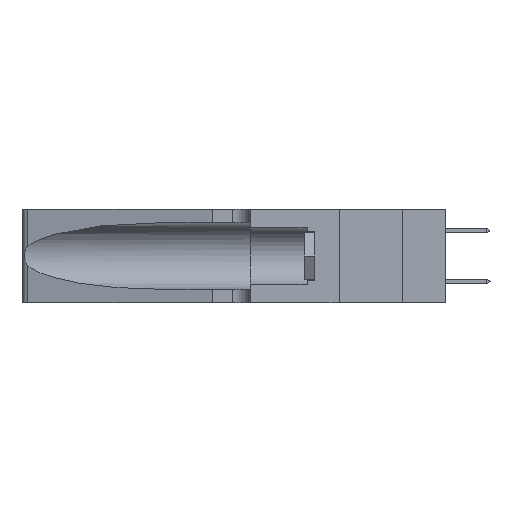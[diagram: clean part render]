
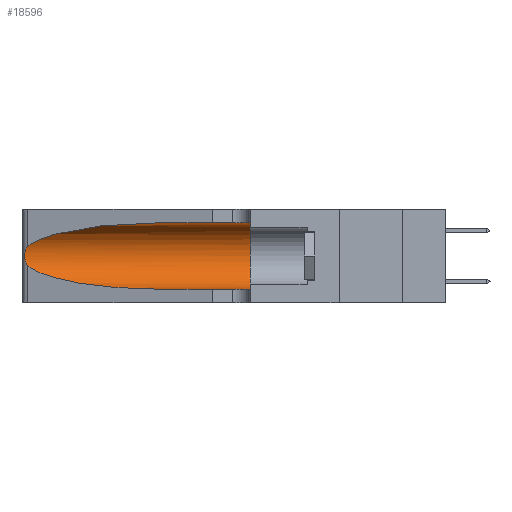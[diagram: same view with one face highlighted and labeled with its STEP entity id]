
A CAD part, left-side view. The second image highlights one B-rep face of the part: STEP entity #18596.
In plain terms, the highlighted cylindrical face has radius 3.308 mm (diameter 6.617 mm), a partial arc.
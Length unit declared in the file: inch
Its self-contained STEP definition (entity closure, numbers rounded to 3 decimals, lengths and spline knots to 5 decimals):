
#35 = AXIS2_PLACEMENT_3D ( 'NONE', #16822, #6896, #2547 ) ;
#482 = CIRCLE ( 'NONE', #35, 0.13025 ) ;
#870 = CARTESIAN_POINT ( 'NONE',  ( 0.25487, 1.22718, 0.14631 ) ) ;
#1161 = VERTEX_POINT ( 'NONE', #9389 ) ;
#1802 = ORIENTED_EDGE ( 'NONE', *, *, #7298, .T. ) ;
#2356 = CARTESIAN_POINT ( 'NONE',  ( 0.18966, 0.96281, 0.31525 ) ) ;
#2547 = DIRECTION ( 'NONE',  ( 0., 0., 1. ) ) ;
#2928 = CARTESIAN_POINT ( 'NONE',  ( 0.25789, 1.23486, 0.15765 ) ) ;
#2979 = CARTESIAN_POINT ( 'NONE',  ( 0.1305, 0.72297, 0.31525 ) ) ;
#3035 = CARTESIAN_POINT ( 'NONE',  ( 0.25487, 1.22718, 0.14631 ) ) ;
#3127 = CYLINDRICAL_SURFACE ( 'NONE', #32522, 0.13025 ) ;
#4473 = CARTESIAN_POINT ( 'NONE',  ( 0.1305, 1.61858, 0.31525 ) ) ;
#5204 = EDGE_CURVE ( 'NONE', #24129, #1161, #13698, .T. ) ;
#5272 = CARTESIAN_POINT ( 'NONE',  ( 0.1305, 0.35, 0.31525 ) ) ;
#5570 = CARTESIAN_POINT ( 'NONE',  ( 0.25639, 1.23184, 0.21858 ) ) ;
#6896 = DIRECTION ( 'NONE',  ( 0., 1., 0. ) ) ;
#7298 = EDGE_CURVE ( 'NONE', #15252, #26612, #16400, .T. ) ;
#7768 = EDGE_CURVE ( 'NONE', #15252, #15232, #14858, .T. ) ;
#7951 = CARTESIAN_POINT ( 'NONE',  ( 0.1305, 0.72297, 0.31525 ) ) ;
#8171 = CARTESIAN_POINT ( 'NONE',  ( 0.25639, 1.23186, 0.15144 ) ) ;
#8453 = CARTESIAN_POINT ( 'NONE',  ( 0.26075, 1.23896, 0.178 ) ) ;
#9302 = DIRECTION ( 'NONE',  ( 0., 0., -1. ) ) ;
#9389 = CARTESIAN_POINT ( 'NONE',  ( 0.1305, 0.35, 0.05475 ) ) ;
#9943 = ORIENTED_EDGE ( 'NONE', *, *, #29032, .T. ) ;
#10994 = CARTESIAN_POINT ( 'NONE',  ( 0.25854, 1.2359, 0.20912 ) ) ;
#11046 = EDGE_CURVE ( 'NONE', #15232, #1161, #482, .T. ) ;
#11238 = CARTESIAN_POINT ( 'NONE',  ( 0.25487, 1.22718, 0.22369 ) ) ;
#11675 = VECTOR ( 'NONE', #27186, 39.37008 ) ;
#11795 = B_SPLINE_CURVE_WITH_KNOTS ( 'NONE', 3,
 ( #13508, #31803, #5570, #21675, #10994, #26729, #24198, #8453, #31702, #15930, #2928, #8171, #29154, #3035 ),
 .UNSPECIFIED., .F., .F.,
 ( 4, 2, 2, 2, 2, 2, 4 ),
 ( 0., 0.00027, 0.00053, 0.00107, 0.0016, 0.00187, 0.00214 ),
 .UNSPECIFIED. ) ;
#12964 = CARTESIAN_POINT ( 'NONE',  ( 0.2373, 1.15595, 0.28018 ) ) ;
#13508 = CARTESIAN_POINT ( 'NONE',  ( 0.25487, 1.22718, 0.22369 ) ) ;
#13698 = LINE ( 'NONE', #13721, #11675 ) ;
#13721 = CARTESIAN_POINT ( 'NONE',  ( 0.1305, 1.61858, 0.05475 ) ) ;
#14858 = LINE ( 'NONE', #4473, #19383 ) ;
#14935 = DIRECTION ( 'NONE',  ( 0., -1., 0. ) ) ;
#14974 =( BOUNDED_CURVE ( )  B_SPLINE_CURVE ( 3, ( #870, #32442, #29368, #21584 ),
 .UNSPECIFIED., .F., .T. ) 
 B_SPLINE_CURVE_WITH_KNOTS ( ( 4, 4 ),
 ( 3.44316, 4.71239 ),
 .UNSPECIFIED. ) 
 CURVE ( )  GEOMETRIC_REPRESENTATION_ITEM ( )  RATIONAL_B_SPLINE_CURVE ( ( 1., 0.87, 0.87, 1. ) ) 
 REPRESENTATION_ITEM ( '' )  );
#15232 = VERTEX_POINT ( 'NONE', #5272 ) ;
#15252 = VERTEX_POINT ( 'NONE', #2979 ) ;
#15535 = FACE_OUTER_BOUND ( 'NONE', #16329, .T. ) ;
#15930 = CARTESIAN_POINT ( 'NONE',  ( 0.25856, 1.23593, 0.16098 ) ) ;
#16329 = EDGE_LOOP ( 'NONE', ( #1802, #9943, #26717, #25968, #26990, #27705 ) ) ;
#16400 =( BOUNDED_CURVE ( )  B_SPLINE_CURVE ( 3, ( #7951, #2356, #12964, #21028 ),
 .UNSPECIFIED., .F., .T. ) 
 B_SPLINE_CURVE_WITH_KNOTS ( ( 4, 4 ),
 ( 1.5708, 2.84003 ),
 .UNSPECIFIED. ) 
 CURVE ( )  GEOMETRIC_REPRESENTATION_ITEM ( )  RATIONAL_B_SPLINE_CURVE ( ( 1., 0.87, 0.87, 1. ) ) 
 REPRESENTATION_ITEM ( '' )  );
#16822 = CARTESIAN_POINT ( 'NONE',  ( 0.1305, 0.35, 0.185 ) ) ;
#18596 = ADVANCED_FACE ( 'NONE', ( #15535 ), #3127, .F. ) ;
#19383 = VECTOR ( 'NONE', #14935, 39.37008 ) ;
#20105 = DIRECTION ( 'NONE',  ( 0., -1., 0. ) ) ;
#21028 = CARTESIAN_POINT ( 'NONE',  ( 0.25487, 1.22718, 0.22369 ) ) ;
#21372 = CARTESIAN_POINT ( 'NONE',  ( 0.25487, 1.22718, 0.14631 ) ) ;
#21584 = CARTESIAN_POINT ( 'NONE',  ( 0.1305, 0.72297, 0.05475 ) ) ;
#21675 = CARTESIAN_POINT ( 'NONE',  ( 0.25787, 1.23484, 0.2124 ) ) ;
#22385 = CARTESIAN_POINT ( 'NONE',  ( 0.1305, 1.61858, 0.185 ) ) ;
#23313 = CARTESIAN_POINT ( 'NONE',  ( 0.1305, 0.72297, 0.05475 ) ) ;
#24129 = VERTEX_POINT ( 'NONE', #23313 ) ;
#24198 = CARTESIAN_POINT ( 'NONE',  ( 0.26075, 1.23896, 0.19203 ) ) ;
#25556 = VERTEX_POINT ( 'NONE', #21372 ) ;
#25754 = EDGE_CURVE ( 'NONE', #25556, #24129, #14974, .T. ) ;
#25968 = ORIENTED_EDGE ( 'NONE', *, *, #5204, .T. ) ;
#26612 = VERTEX_POINT ( 'NONE', #11238 ) ;
#26717 = ORIENTED_EDGE ( 'NONE', *, *, #25754, .T. ) ;
#26729 = CARTESIAN_POINT ( 'NONE',  ( 0.26018, 1.23835, 0.19895 ) ) ;
#26990 = ORIENTED_EDGE ( 'NONE', *, *, #11046, .F. ) ;
#27186 = DIRECTION ( 'NONE',  ( 0., -1., 0. ) ) ;
#27705 = ORIENTED_EDGE ( 'NONE', *, *, #7768, .F. ) ;
#29032 = EDGE_CURVE ( 'NONE', #26612, #25556, #11795, .T. ) ;
#29154 = CARTESIAN_POINT ( 'NONE',  ( 0.25555, 1.22993, 0.14849 ) ) ;
#29368 = CARTESIAN_POINT ( 'NONE',  ( 0.18966, 0.96281, 0.05475 ) ) ;
#31702 = CARTESIAN_POINT ( 'NONE',  ( 0.26017, 1.23833, 0.17102 ) ) ;
#31803 = CARTESIAN_POINT ( 'NONE',  ( 0.25555, 1.22994, 0.2215 ) ) ;
#32442 = CARTESIAN_POINT ( 'NONE',  ( 0.2373, 1.15595, 0.08982 ) ) ;
#32522 = AXIS2_PLACEMENT_3D ( 'NONE', #22385, #20105, #9302 ) ;
